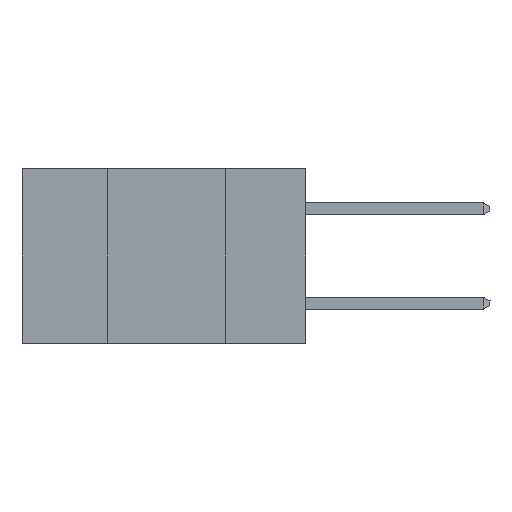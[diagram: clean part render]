
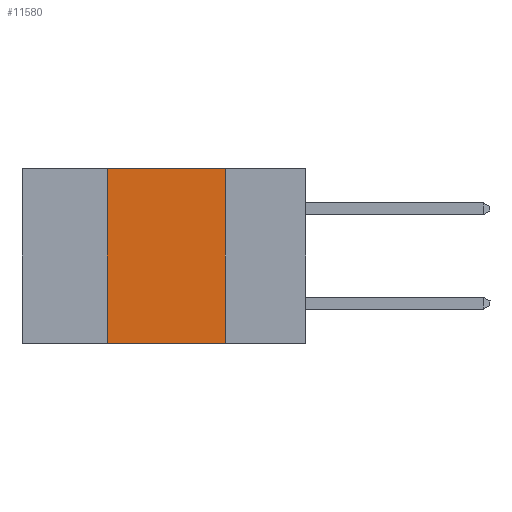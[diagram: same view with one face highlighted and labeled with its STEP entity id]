
A CAD part, left-side view. The second image highlights one B-rep face of the part: STEP entity #11580.
In plain terms, the highlighted planar face has unit normal (-1, 0, 0).
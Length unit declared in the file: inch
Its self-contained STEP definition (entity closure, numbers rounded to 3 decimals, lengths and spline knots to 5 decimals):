
#37 = VERTEX_POINT ( 'NONE', #4866 ) ;
#365 = EDGE_CURVE ( 'NONE', #5095, #9092, #2129, .T. ) ;
#522 = ORIENTED_EDGE ( 'NONE', *, *, #6822, .F. ) ;
#693 = VECTOR ( 'NONE', #3765, 39.37008 ) ;
#975 = DIRECTION ( 'NONE',  ( 1., 0., 0. ) ) ;
#994 = CARTESIAN_POINT ( 'NONE',  ( 0., 0.42, -0.37 ) ) ;
#1125 = ORIENTED_EDGE ( 'NONE', *, *, #6107, .F. ) ;
#1750 = AXIS2_PLACEMENT_3D ( 'NONE', #7408, #975, #8863 ) ;
#2129 = LINE ( 'NONE', #12197, #693 ) ;
#2934 = FACE_OUTER_BOUND ( 'NONE', #3543, .T. ) ;
#3267 = VECTOR ( 'NONE', #6169, 39.37008 ) ;
#3543 = EDGE_LOOP ( 'NONE', ( #1125, #12810, #522, #12013 ) ) ;
#3765 = DIRECTION ( 'NONE',  ( 0., -1., 0. ) ) ;
#4689 = VECTOR ( 'NONE', #14462, 39.37008 ) ;
#4866 = CARTESIAN_POINT ( 'NONE',  ( 0., 0.17, 0. ) ) ;
#5095 = VERTEX_POINT ( 'NONE', #994 ) ;
#6107 = EDGE_CURVE ( 'NONE', #37, #9092, #11269, .T. ) ;
#6169 = DIRECTION ( 'NONE',  ( 0., -1., 0. ) ) ;
#6282 = PLANE ( 'NONE',  #1750 ) ;
#6698 = CARTESIAN_POINT ( 'NONE',  ( 0., 0.42, 0. ) ) ;
#6822 = EDGE_CURVE ( 'NONE', #5095, #15724, #10487, .T. ) ;
#7252 = VECTOR ( 'NONE', #12993, 39.37008 ) ;
#7408 = CARTESIAN_POINT ( 'NONE',  ( 0., 0.6, 0. ) ) ;
#8020 = CARTESIAN_POINT ( 'NONE',  ( 0., 0.42, 0. ) ) ;
#8863 = DIRECTION ( 'NONE',  ( 0., 0., -1. ) ) ;
#9092 = VERTEX_POINT ( 'NONE', #10545 ) ;
#10487 = LINE ( 'NONE', #8020, #4689 ) ;
#10503 = CARTESIAN_POINT ( 'NONE',  ( 0., 0.17, 0. ) ) ;
#10545 = CARTESIAN_POINT ( 'NONE',  ( 0., 0.17, -0.37 ) ) ;
#11269 = LINE ( 'NONE', #10503, #7252 ) ;
#11580 = ADVANCED_FACE ( 'NONE', ( #2934 ), #6282, .F. ) ;
#12013 = ORIENTED_EDGE ( 'NONE', *, *, #365, .T. ) ;
#12197 = CARTESIAN_POINT ( 'NONE',  ( 0., 0.6, -0.37 ) ) ;
#12810 = ORIENTED_EDGE ( 'NONE', *, *, #14489, .F. ) ;
#12993 = DIRECTION ( 'NONE',  ( 0., 0., -1. ) ) ;
#14128 = LINE ( 'NONE', #15078, #3267 ) ;
#14462 = DIRECTION ( 'NONE',  ( 0., 0., 1. ) ) ;
#14489 = EDGE_CURVE ( 'NONE', #15724, #37, #14128, .T. ) ;
#15078 = CARTESIAN_POINT ( 'NONE',  ( 0., 0.6, 0. ) ) ;
#15724 = VERTEX_POINT ( 'NONE', #6698 ) ;
